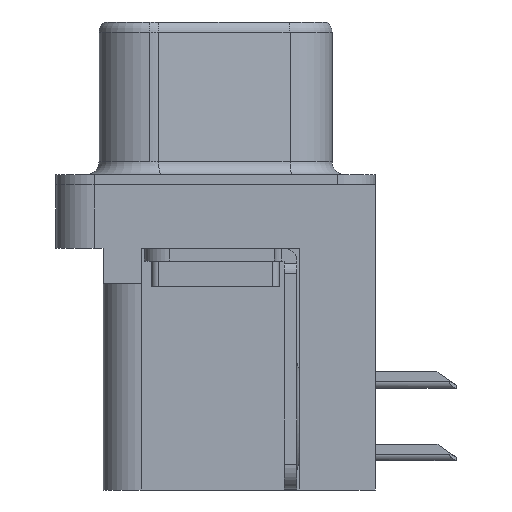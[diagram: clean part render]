
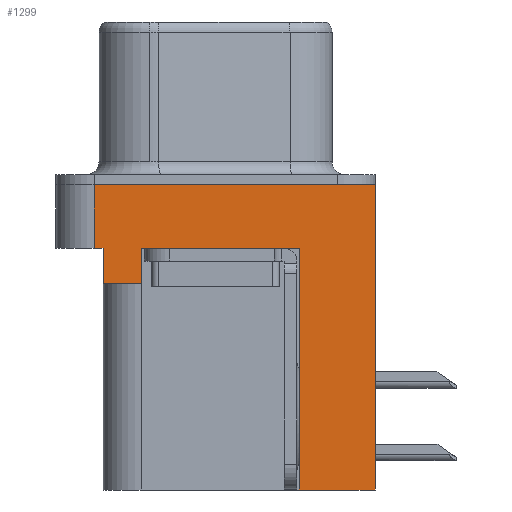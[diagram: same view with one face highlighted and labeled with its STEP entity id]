
A CAD part, left-side view. The second image highlights one B-rep face of the part: STEP entity #1299.
In plain terms, the highlighted planar face has unit normal (-1, 0, 0).
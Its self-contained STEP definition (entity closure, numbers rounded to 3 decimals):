
#58 = VERTEX_POINT ( 'NONE', #6948 ) ;
#534 = CARTESIAN_POINT ( 'NONE',  ( -2.91, 4.425, -3.9 ) ) ;
#631 = CARTESIAN_POINT ( 'NONE',  ( -2.91, -3.295, -12. ) ) ;
#705 = ORIENTED_EDGE ( 'NONE', *, *, #10998, .T. ) ;
#1006 = CARTESIAN_POINT ( 'NONE',  ( -2.91, 4.775, -2.5 ) ) ;
#1299 = ADVANCED_FACE ( 'NONE', ( #13479 ), #10273, .T. ) ;
#1302 = CARTESIAN_POINT ( 'NONE',  ( -2.91, -6.275, -2.5 ) ) ;
#1374 = VERTEX_POINT ( 'NONE', #10528 ) ;
#1647 = CARTESIAN_POINT ( 'NONE',  ( -2.91, -3.295, -12. ) ) ;
#1829 = ORIENTED_EDGE ( 'NONE', *, *, #13994, .F. ) ;
#1992 = EDGE_CURVE ( 'NONE', #2683, #2386, #14227, .T. ) ;
#2009 = ORIENTED_EDGE ( 'NONE', *, *, #3746, .F. ) ;
#2036 = DIRECTION ( 'NONE',  ( 0., 0., 1. ) ) ;
#2218 = VECTOR ( 'NONE', #15315, 1000. ) ;
#2278 = LINE ( 'NONE', #534, #6111 ) ;
#2386 = VERTEX_POINT ( 'NONE', #6279 ) ;
#2495 = VERTEX_POINT ( 'NONE', #14248 ) ;
#2623 = LINE ( 'NONE', #13575, #14091 ) ;
#2683 = VERTEX_POINT ( 'NONE', #7029 ) ;
#2855 = DIRECTION ( 'NONE',  ( 0., 1., 0. ) ) ;
#3746 = EDGE_CURVE ( 'NONE', #1374, #9121, #15048, .T. ) ;
#3751 = VECTOR ( 'NONE', #6095, 1000. ) ;
#3916 = LINE ( 'NONE', #11006, #12320 ) ;
#4352 = CARTESIAN_POINT ( 'NONE',  ( -2.91, 4.425, -3.9 ) ) ;
#4591 = CARTESIAN_POINT ( 'NONE',  ( -2.91, 4.425, -3.9 ) ) ;
#5306 = CARTESIAN_POINT ( 'NONE',  ( -2.91, -6.275, -2.5 ) ) ;
#5352 = DIRECTION ( 'NONE',  ( 0., 0., 1. ) ) ;
#5903 = ORIENTED_EDGE ( 'NONE', *, *, #1992, .T. ) ;
#5914 = ORIENTED_EDGE ( 'NONE', *, *, #9125, .F. ) ;
#6048 = VECTOR ( 'NONE', #15604, 1000. ) ;
#6095 = DIRECTION ( 'NONE',  ( 0., -1., 0. ) ) ;
#6111 = VECTOR ( 'NONE', #9178, 1000. ) ;
#6279 = CARTESIAN_POINT ( 'NONE',  ( -2.91, 2.895, -2.5 ) ) ;
#6835 = LINE ( 'NONE', #15203, #12380 ) ;
#6948 = CARTESIAN_POINT ( 'NONE',  ( -2.91, -3.295, -2.5 ) ) ;
#7029 = CARTESIAN_POINT ( 'NONE',  ( -2.91, 2.895, -3.9 ) ) ;
#7112 = ORIENTED_EDGE ( 'NONE', *, *, #14374, .T. ) ;
#7170 = DIRECTION ( 'NONE',  ( 0., 0., 1. ) ) ;
#7660 = ORIENTED_EDGE ( 'NONE', *, *, #10837, .F. ) ;
#7712 = VECTOR ( 'NONE', #2036, 1000. ) ;
#7757 = LINE ( 'NONE', #1006, #6048 ) ;
#7944 = CARTESIAN_POINT ( 'NONE',  ( -2.91, 4.425, -2.5 ) ) ;
#8074 = ORIENTED_EDGE ( 'NONE', *, *, #14697, .F. ) ;
#8279 = EDGE_LOOP ( 'NONE', ( #7660, #15745, #9595, #1829, #5914, #5903, #705, #8074, #2009, #7112 ) ) ;
#8449 = VERTEX_POINT ( 'NONE', #11486 ) ;
#8561 = VERTEX_POINT ( 'NONE', #11540 ) ;
#8912 = LINE ( 'NONE', #1302, #3751 ) ;
#8942 = DIRECTION ( 'NONE',  ( 0., -1., 0. ) ) ;
#9121 = VERTEX_POINT ( 'NONE', #631 ) ;
#9125 = EDGE_CURVE ( 'NONE', #2683, #12990, #2278, .T. ) ;
#9178 = DIRECTION ( 'NONE',  ( 0., 1., 0. ) ) ;
#9339 = CARTESIAN_POINT ( 'NONE',  ( -2.91, 2.895, -3.9 ) ) ;
#9595 = ORIENTED_EDGE ( 'NONE', *, *, #12498, .T. ) ;
#10273 = PLANE ( 'NONE',  #12527 ) ;
#10528 = CARTESIAN_POINT ( 'NONE',  ( -2.91, -6.275, -12. ) ) ;
#10837 = EDGE_CURVE ( 'NONE', #2495, #8449, #2623, .T. ) ;
#10998 = EDGE_CURVE ( 'NONE', #2386, #58, #6835, .T. ) ;
#11006 = CARTESIAN_POINT ( 'NONE',  ( -2.91, -6.275, -2.5 ) ) ;
#11486 = CARTESIAN_POINT ( 'NONE',  ( -2.91, -6.275, 0. ) ) ;
#11540 = CARTESIAN_POINT ( 'NONE',  ( -2.91, 4.775, -2.5 ) ) ;
#11746 = DIRECTION ( 'NONE',  ( 0., 0., 1. ) ) ;
#11772 = VECTOR ( 'NONE', #2855, 1000. ) ;
#12023 = EDGE_CURVE ( 'NONE', #8561, #2495, #7757, .T. ) ;
#12320 = VECTOR ( 'NONE', #7170, 1000. ) ;
#12380 = VECTOR ( 'NONE', #8942, 1000. ) ;
#12498 = EDGE_CURVE ( 'NONE', #8561, #13418, #8912, .T. ) ;
#12527 = AXIS2_PLACEMENT_3D ( 'NONE', #5306, #13900, #5352 ) ;
#12889 = LINE ( 'NONE', #15253, #13067 ) ;
#12990 = VERTEX_POINT ( 'NONE', #4591 ) ;
#13067 = VECTOR ( 'NONE', #11746, 1000. ) ;
#13418 = VERTEX_POINT ( 'NONE', #7944 ) ;
#13479 = FACE_OUTER_BOUND ( 'NONE', #8279, .T. ) ;
#13575 = CARTESIAN_POINT ( 'NONE',  ( -2.91, -6.275, 0. ) ) ;
#13900 = DIRECTION ( 'NONE',  ( -1., 0., 0. ) ) ;
#13994 = EDGE_CURVE ( 'NONE', #12990, #13418, #15799, .T. ) ;
#14091 = VECTOR ( 'NONE', #14717, 1000. ) ;
#14227 = LINE ( 'NONE', #9339, #7712 ) ;
#14248 = CARTESIAN_POINT ( 'NONE',  ( -2.91, 4.775, 0. ) ) ;
#14374 = EDGE_CURVE ( 'NONE', #1374, #8449, #3916, .T. ) ;
#14697 = EDGE_CURVE ( 'NONE', #9121, #58, #12889, .T. ) ;
#14717 = DIRECTION ( 'NONE',  ( 0., -1., 0. ) ) ;
#15048 = LINE ( 'NONE', #1647, #11772 ) ;
#15203 = CARTESIAN_POINT ( 'NONE',  ( -2.91, -6.275, -2.5 ) ) ;
#15253 = CARTESIAN_POINT ( 'NONE',  ( -2.91, -3.295, -12. ) ) ;
#15315 = DIRECTION ( 'NONE',  ( 0., 0., 1. ) ) ;
#15604 = DIRECTION ( 'NONE',  ( 0., 0., 1. ) ) ;
#15745 = ORIENTED_EDGE ( 'NONE', *, *, #12023, .F. ) ;
#15799 = LINE ( 'NONE', #4352, #2218 ) ;
